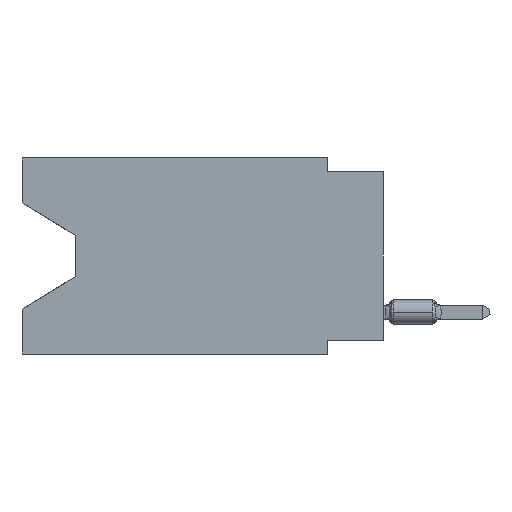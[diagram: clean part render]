
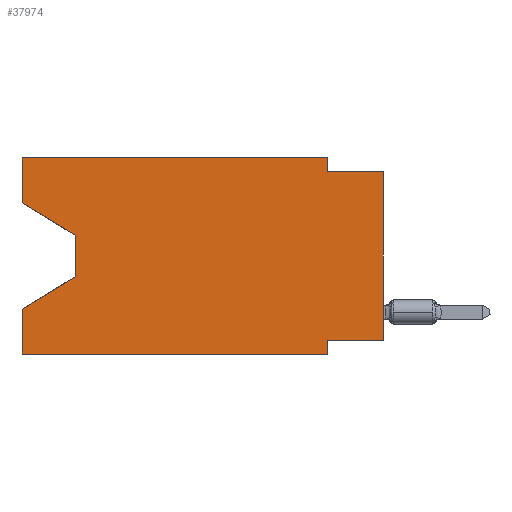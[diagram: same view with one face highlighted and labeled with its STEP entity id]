
A CAD part, left-side view. The second image highlights one B-rep face of the part: STEP entity #37974.
In plain terms, the highlighted planar face has unit normal (-1, 0, 0).
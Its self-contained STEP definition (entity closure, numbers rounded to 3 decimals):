
#55 = EDGE_CURVE ( 'NONE', #30552, #73408, #1485, .T. ) ;
#443 = LINE ( 'NONE', #14406, #52178 ) ;
#906 = VERTEX_POINT ( 'NONE', #70168 ) ;
#1485 = LINE ( 'NONE', #28968, #16119 ) ;
#4584 = VECTOR ( 'NONE', #80834, 1000. ) ;
#4747 = DIRECTION ( 'NONE',  ( 0., -1., 0. ) ) ;
#5214 = VERTEX_POINT ( 'NONE', #80694 ) ;
#5374 = DIRECTION ( 'NONE',  ( 0., -1., 0. ) ) ;
#5444 = ORIENTED_EDGE ( 'NONE', *, *, #51399, .T. ) ;
#5966 = VECTOR ( 'NONE', #10769, 1000. ) ;
#7177 = VECTOR ( 'NONE', #17848, 1000. ) ;
#10328 = ORIENTED_EDGE ( 'NONE', *, *, #10829, .F. ) ;
#10769 = DIRECTION ( 'NONE',  ( 0., -1., 0. ) ) ;
#10829 = EDGE_CURVE ( 'NONE', #906, #5214, #24603, .T. ) ;
#11078 = CARTESIAN_POINT ( 'NONE',  ( 0., 13.97, -5.385 ) ) ;
#11521 = CARTESIAN_POINT ( 'NONE',  ( 0., 0., -0.635 ) ) ;
#11527 = CARTESIAN_POINT ( 'NONE',  ( 0., 16.383, -8.89 ) ) ;
#12160 = VECTOR ( 'NONE', #73253, 1000. ) ;
#13909 = VERTEX_POINT ( 'NONE', #46050 ) ;
#14391 = CARTESIAN_POINT ( 'NONE',  ( 0., 2.54, 0. ) ) ;
#14406 = CARTESIAN_POINT ( 'NONE',  ( 0., 0., -8.255 ) ) ;
#15219 = CARTESIAN_POINT ( 'NONE',  ( 0., 13.97, -3.505 ) ) ;
#16119 = VECTOR ( 'NONE', #81650, 1000. ) ;
#17848 = DIRECTION ( 'NONE',  ( 0., 0., 1. ) ) ;
#21262 = EDGE_CURVE ( 'NONE', #13909, #43144, #65959, .T. ) ;
#21977 = LINE ( 'NONE', #76941, #32577 ) ;
#23244 = ORIENTED_EDGE ( 'NONE', *, *, #76024, .F. ) ;
#24205 = EDGE_CURVE ( 'NONE', #5214, #30552, #31070, .T. ) ;
#24603 = LINE ( 'NONE', #87173, #7177 ) ;
#24947 = VECTOR ( 'NONE', #38575, 1000. ) ;
#25669 = VECTOR ( 'NONE', #52905, 1000. ) ;
#28968 = CARTESIAN_POINT ( 'NONE',  ( 0., 2.54, 0. ) ) ;
#29227 = VERTEX_POINT ( 'NONE', #57022 ) ;
#29627 = DIRECTION ( 'NONE',  ( 0., 0., -1. ) ) ;
#30552 = VERTEX_POINT ( 'NONE', #14391 ) ;
#30678 = DIRECTION ( 'NONE',  ( 0., 0., -1. ) ) ;
#31070 = LINE ( 'NONE', #86872, #5966 ) ;
#31555 = CARTESIAN_POINT ( 'NONE',  ( 0., 16.383, 0. ) ) ;
#31814 = LINE ( 'NONE', #11521, #74248 ) ;
#32301 = ORIENTED_EDGE ( 'NONE', *, *, #55, .F. ) ;
#32577 = VECTOR ( 'NONE', #42720, 1000. ) ;
#33595 = CARTESIAN_POINT ( 'NONE',  ( 0., 2.54, -0.635 ) ) ;
#37705 = CARTESIAN_POINT ( 'NONE',  ( 0., 16.383, -2.038 ) ) ;
#37861 = FACE_OUTER_BOUND ( 'NONE', #74415, .T. ) ;
#37974 = ADVANCED_FACE ( 'NONE', ( #37861 ), #52271, .F. ) ;
#38575 = DIRECTION ( 'NONE',  ( 0., 0.855, -0.519 ) ) ;
#38675 = CARTESIAN_POINT ( 'NONE',  ( 0., 2.54, -8.255 ) ) ;
#39439 = LINE ( 'NONE', #87592, #4584 ) ;
#39897 = VECTOR ( 'NONE', #5374, 1000. ) ;
#41172 = ORIENTED_EDGE ( 'NONE', *, *, #78536, .F. ) ;
#42720 = DIRECTION ( 'NONE',  ( 0., 0., 1. ) ) ;
#43144 = VERTEX_POINT ( 'NONE', #75155 ) ;
#45185 = ORIENTED_EDGE ( 'NONE', *, *, #52624, .T. ) ;
#46050 = CARTESIAN_POINT ( 'NONE',  ( 0., 0., -8.255 ) ) ;
#46388 = LINE ( 'NONE', #66218, #39897 ) ;
#46839 = VERTEX_POINT ( 'NONE', #59717 ) ;
#49613 = VECTOR ( 'NONE', #29627, 1000. ) ;
#51399 = EDGE_CURVE ( 'NONE', #55607, #46839, #72790, .T. ) ;
#52178 = VECTOR ( 'NONE', #55413, 1000. ) ;
#52271 = PLANE ( 'NONE',  #55184 ) ;
#52506 = EDGE_CURVE ( 'NONE', #58773, #55607, #83662, .T. ) ;
#52624 = EDGE_CURVE ( 'NONE', #906, #58773, #86313, .T. ) ;
#52905 = DIRECTION ( 'NONE',  ( 0., 0., 1. ) ) ;
#54523 = EDGE_CURVE ( 'NONE', #80377, #46839, #21977, .T. ) ;
#55184 = AXIS2_PLACEMENT_3D ( 'NONE', #31555, #78839, #30678 ) ;
#55406 = EDGE_CURVE ( 'NONE', #80377, #29227, #46388, .T. ) ;
#55413 = DIRECTION ( 'NONE',  ( 0., 1., 0. ) ) ;
#55607 = VERTEX_POINT ( 'NONE', #68414 ) ;
#57022 = CARTESIAN_POINT ( 'NONE',  ( 0., 2.54, -8.89 ) ) ;
#58773 = VERTEX_POINT ( 'NONE', #75380 ) ;
#59717 = CARTESIAN_POINT ( 'NONE',  ( 0., 16.383, -6.852 ) ) ;
#60336 = ORIENTED_EDGE ( 'NONE', *, *, #52506, .T. ) ;
#60958 = ORIENTED_EDGE ( 'NONE', *, *, #86837, .F. ) ;
#63566 = ORIENTED_EDGE ( 'NONE', *, *, #24205, .F. ) ;
#65959 = LINE ( 'NONE', #66856, #25669 ) ;
#66218 = CARTESIAN_POINT ( 'NONE',  ( 0., 16.383, -8.89 ) ) ;
#66856 = CARTESIAN_POINT ( 'NONE',  ( 0., 0., 0. ) ) ;
#68414 = CARTESIAN_POINT ( 'NONE',  ( 0., 13.97, -5.385 ) ) ;
#70168 = CARTESIAN_POINT ( 'NONE',  ( 0., 16.383, -2.038 ) ) ;
#70764 = ORIENTED_EDGE ( 'NONE', *, *, #55406, .T. ) ;
#72709 = ORIENTED_EDGE ( 'NONE', *, *, #21262, .T. ) ;
#72790 = LINE ( 'NONE', #11078, #24947 ) ;
#73253 = DIRECTION ( 'NONE',  ( 0., -0.855, -0.519 ) ) ;
#73408 = VERTEX_POINT ( 'NONE', #33595 ) ;
#74248 = VECTOR ( 'NONE', #4747, 1000. ) ;
#74415 = EDGE_LOOP ( 'NONE', ( #45185, #60336, #5444, #76528, #70764, #23244, #41172, #72709, #60958, #32301, #63566, #10328 ) ) ;
#75155 = CARTESIAN_POINT ( 'NONE',  ( 0., 0., -0.635 ) ) ;
#75380 = CARTESIAN_POINT ( 'NONE',  ( 0., 13.97, -3.505 ) ) ;
#76024 = EDGE_CURVE ( 'NONE', #79946, #29227, #39439, .T. ) ;
#76528 = ORIENTED_EDGE ( 'NONE', *, *, #54523, .F. ) ;
#76941 = CARTESIAN_POINT ( 'NONE',  ( 0., 16.383, 0. ) ) ;
#78536 = EDGE_CURVE ( 'NONE', #13909, #79946, #443, .T. ) ;
#78839 = DIRECTION ( 'NONE',  ( 1., 0., 0. ) ) ;
#79946 = VERTEX_POINT ( 'NONE', #38675 ) ;
#80377 = VERTEX_POINT ( 'NONE', #11527 ) ;
#80694 = CARTESIAN_POINT ( 'NONE',  ( 0., 16.383, 0. ) ) ;
#80834 = DIRECTION ( 'NONE',  ( 0., 0., -1. ) ) ;
#81650 = DIRECTION ( 'NONE',  ( 0., 0., -1. ) ) ;
#83662 = LINE ( 'NONE', #15219, #49613 ) ;
#86313 = LINE ( 'NONE', #37705, #12160 ) ;
#86837 = EDGE_CURVE ( 'NONE', #73408, #43144, #31814, .T. ) ;
#86872 = CARTESIAN_POINT ( 'NONE',  ( 0., 16.383, 0. ) ) ;
#87173 = CARTESIAN_POINT ( 'NONE',  ( 0., 16.383, 0. ) ) ;
#87592 = CARTESIAN_POINT ( 'NONE',  ( 0., 2.54, -8.89 ) ) ;
